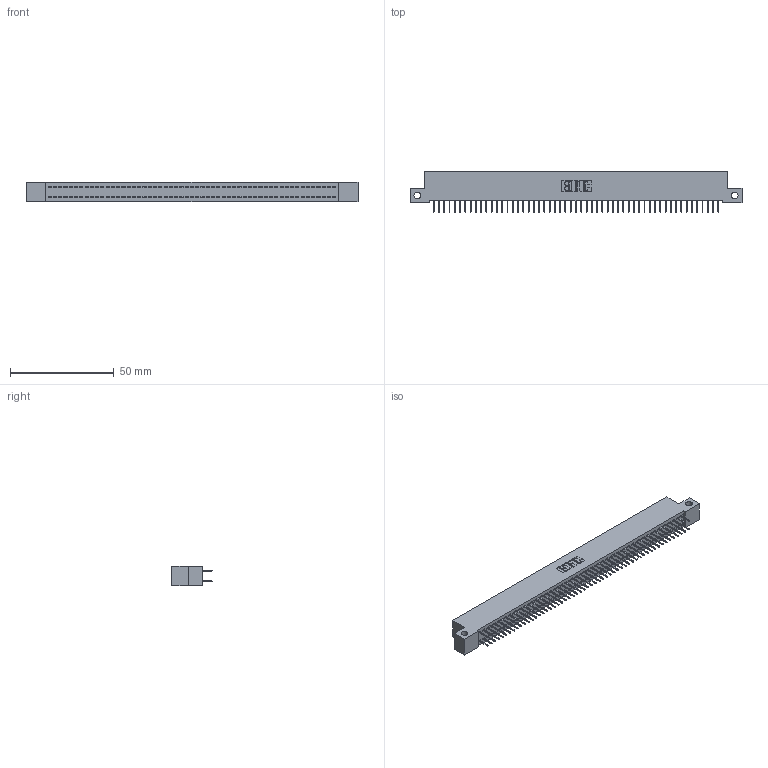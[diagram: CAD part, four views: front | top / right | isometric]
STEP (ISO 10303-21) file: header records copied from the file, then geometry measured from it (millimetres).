
FILE_DESCRIPTION (( 'STEP AP203' ), '1' );
FILE_NAME ('392-110-524-212.STEP', '2018-08-18T21:40:08', ( '' ), ( '' ), 'SwSTEP 2.0', 'SolidWorks 2016', '' );
FILE_SCHEMA (( 'CONFIG_CONTROL_DESIGN' ));
Length unit declared in the file: inch
Products named in the file (3): 392-110-524-212; 342 Part_Side Mount; 345-292-001_345-293-124
Assembly tree (111 placements, depth 2):
  392-110-524-212
    342 Part_Side Mount
    345-292-001_345-293-124  x110
Bounding box: 160.02 x 19.69 x 9.4 mm (x, y, z)
Volume: 14198.9 mm3; surface area: 22839.8 mm2
Topology: 111 solids, 111 shells, 6270 faces, 17789 edges, 11418 vertices
Faces by surface type: plane 4686, cylinder 1584
Entity records: 33647 total; most frequent: CARTESIAN_POINT 5558, ORIENTED_EDGE 5494, DIRECTION 4727, EDGE_CURVE 2747, VECTOR 2623, LINE 2623, VERTEX_POINT 1826, AXIS2_PLACEMENT_3D 1052
